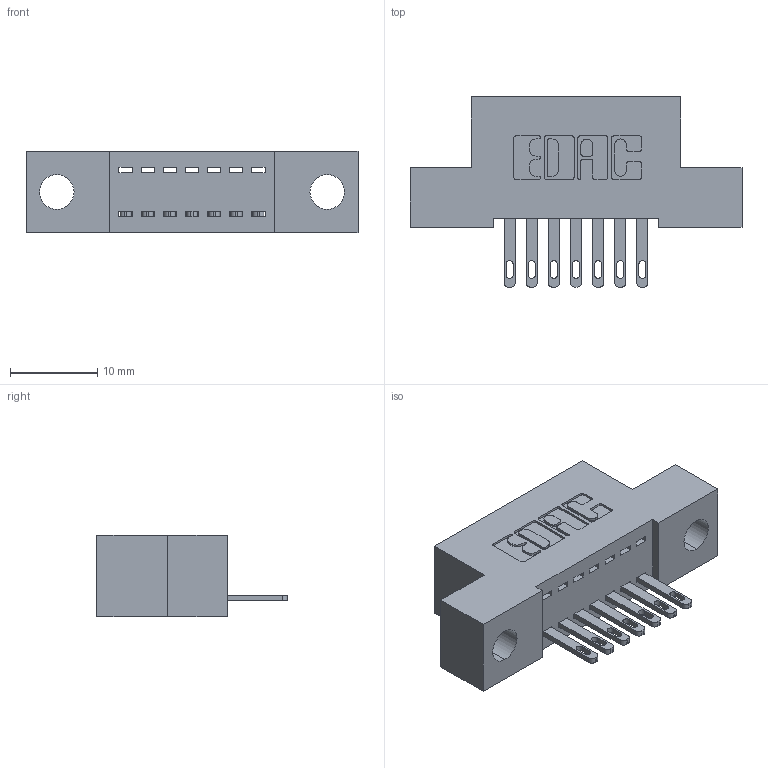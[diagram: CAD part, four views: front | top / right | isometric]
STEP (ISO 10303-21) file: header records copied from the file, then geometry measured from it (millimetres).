
FILE_DESCRIPTION (( 'STEP AP203' ), '1' );
FILE_NAME ('342-007-500-104.STEP', '2019-10-01T12:42:32', ( '' ), ( '' ), 'SwSTEP 2.0', 'SolidWorks 2016', '' );
FILE_SCHEMA (( 'CONFIG_CONTROL_DESIGN' ));
Length unit declared in the file: inch
Products named in the file (3): 342 Part_.156 TH; 345-292-001_345-293-100; 342-007-500-104
Assembly tree (8 placements, depth 2):
  342-007-500-104
    342 Part_.156 TH
    345-292-001_345-293-100  x7
Bounding box: 38.1 x 21.85 x 9.4 mm (x, y, z)
Volume: 3129 mm3; surface area: 3773.9 mm2
Topology: 8 solids, 8 shells, 488 faces, 1475 edges, 982 vertices
Faces by surface type: plane 318, cylinder 170
Entity records: 8607 total; most frequent: CARTESIAN_POINT 1495, ORIENTED_EDGE 1438, DIRECTION 1333, EDGE_CURVE 719, LINE 587, VECTOR 587, VERTEX_POINT 478, AXIS2_PLACEMENT_3D 373
